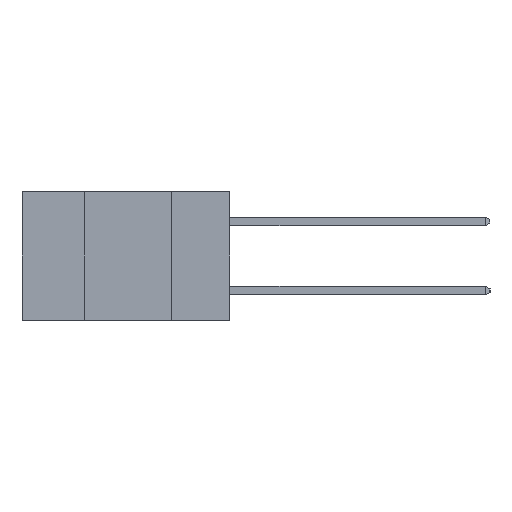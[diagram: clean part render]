
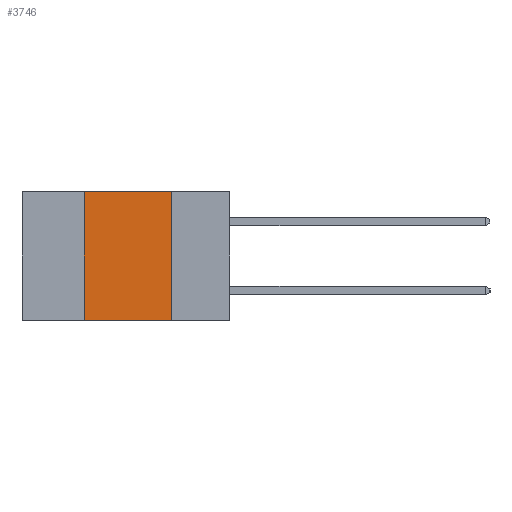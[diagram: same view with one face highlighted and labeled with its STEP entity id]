
A CAD part, left-side view. The second image highlights one B-rep face of the part: STEP entity #3746.
In plain terms, the highlighted planar face has unit normal (-1, 0, 0).
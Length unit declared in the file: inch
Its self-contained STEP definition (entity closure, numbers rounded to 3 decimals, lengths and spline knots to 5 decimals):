
#273 = CARTESIAN_POINT ( 'NONE',  ( 0., 0.42, -0.37 ) ) ;
#658 = CARTESIAN_POINT ( 'NONE',  ( 0., 0.17, -0.37 ) ) ;
#713 = EDGE_CURVE ( 'NONE', #3976, #11769, #8301, .T. ) ;
#1604 = LINE ( 'NONE', #11363, #4729 ) ;
#2106 = EDGE_LOOP ( 'NONE', ( #7857, #7893, #7992, #8404 ) ) ;
#2677 = DIRECTION ( 'NONE',  ( 0., 0., -1. ) ) ;
#2747 = DIRECTION ( 'NONE',  ( 1., 0., 0. ) ) ;
#2772 = PLANE ( 'NONE',  #6953 ) ;
#2838 = CARTESIAN_POINT ( 'NONE',  ( 0., 0.6, 0. ) ) ;
#2975 = DIRECTION ( 'NONE',  ( 0., -1., 0. ) ) ;
#3181 = EDGE_CURVE ( 'NONE', #3976, #8037, #1604, .T. ) ;
#3746 = ADVANCED_FACE ( 'NONE', ( #5403 ), #2772, .F. ) ;
#3832 = DIRECTION ( 'NONE',  ( 0., 0., -1. ) ) ;
#3844 = CARTESIAN_POINT ( 'NONE',  ( 0., 0.17, -0.37 ) ) ;
#3976 = VERTEX_POINT ( 'NONE', #273 ) ;
#4729 = VECTOR ( 'NONE', #11343, 39.37008 ) ;
#4792 = CARTESIAN_POINT ( 'NONE',  ( 0., 0.17, 0. ) ) ;
#5153 = LINE ( 'NONE', #3844, #12860 ) ;
#5403 = FACE_OUTER_BOUND ( 'NONE', #2106, .T. ) ;
#5444 = EDGE_CURVE ( 'NONE', #8037, #11210, #10342, .T. ) ;
#6910 = EDGE_CURVE ( 'NONE', #11210, #11769, #5153, .T. ) ;
#6953 = AXIS2_PLACEMENT_3D ( 'NONE', #2838, #2747, #2677 ) ;
#7565 = VECTOR ( 'NONE', #12059, 39.37008 ) ;
#7857 = ORIENTED_EDGE ( 'NONE', *, *, #6910, .F. ) ;
#7893 = ORIENTED_EDGE ( 'NONE', *, *, #5444, .F. ) ;
#7992 = ORIENTED_EDGE ( 'NONE', *, *, #3181, .F. ) ;
#8037 = VERTEX_POINT ( 'NONE', #12244 ) ;
#8301 = LINE ( 'NONE', #12915, #10937 ) ;
#8404 = ORIENTED_EDGE ( 'NONE', *, *, #713, .T. ) ;
#10342 = LINE ( 'NONE', #12147, #7565 ) ;
#10937 = VECTOR ( 'NONE', #2975, 39.37008 ) ;
#11210 = VERTEX_POINT ( 'NONE', #4792 ) ;
#11343 = DIRECTION ( 'NONE',  ( 0., 0., 1. ) ) ;
#11363 = CARTESIAN_POINT ( 'NONE',  ( 0., 0.42, -0.37 ) ) ;
#11769 = VERTEX_POINT ( 'NONE', #658 ) ;
#12059 = DIRECTION ( 'NONE',  ( 0., -1., 0. ) ) ;
#12147 = CARTESIAN_POINT ( 'NONE',  ( 0., 0.6, 0. ) ) ;
#12244 = CARTESIAN_POINT ( 'NONE',  ( 0., 0.42, 0. ) ) ;
#12860 = VECTOR ( 'NONE', #3832, 39.37008 ) ;
#12915 = CARTESIAN_POINT ( 'NONE',  ( 0., 0.6, -0.37 ) ) ;
